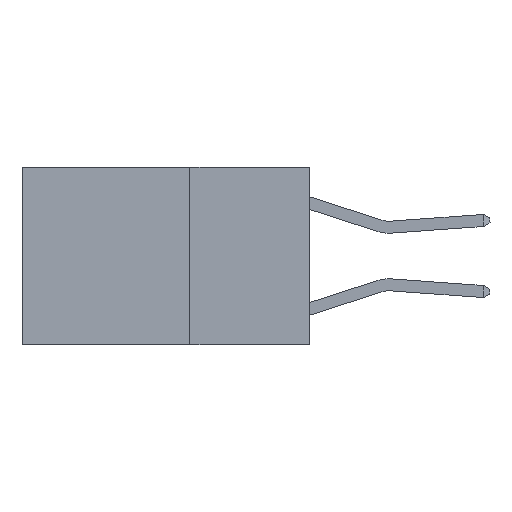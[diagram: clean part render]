
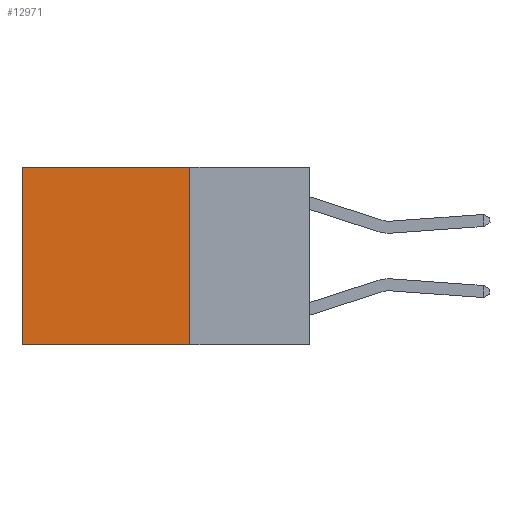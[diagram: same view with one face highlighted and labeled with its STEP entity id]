
A CAD part, left-side view. The second image highlights one B-rep face of the part: STEP entity #12971.
In plain terms, the highlighted planar face has unit normal (-1, 0, 0).
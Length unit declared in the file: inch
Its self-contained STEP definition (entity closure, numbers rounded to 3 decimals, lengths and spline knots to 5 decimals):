
#613 = VECTOR ( 'NONE', #1152, 39.37008 ) ;
#1152 = DIRECTION ( 'NONE',  ( 0., 1., 0. ) ) ;
#1472 = VECTOR ( 'NONE', #15156, 39.37008 ) ;
#1720 = DIRECTION ( 'NONE',  ( 1., 0., 0. ) ) ;
#2119 = VERTEX_POINT ( 'NONE', #9985 ) ;
#2372 = ORIENTED_EDGE ( 'NONE', *, *, #3028, .F. ) ;
#3028 = EDGE_CURVE ( 'NONE', #2119, #4737, #8661, .T. ) ;
#3346 = AXIS2_PLACEMENT_3D ( 'NONE', #12915, #1720, #12985 ) ;
#3936 = ORIENTED_EDGE ( 'NONE', *, *, #6628, .F. ) ;
#4737 = VERTEX_POINT ( 'NONE', #15641 ) ;
#5472 = CARTESIAN_POINT ( 'NONE',  ( 0.2625, 0.25, 0. ) ) ;
#5531 = VERTEX_POINT ( 'NONE', #11012 ) ;
#5959 = VECTOR ( 'NONE', #7079, 39.37008 ) ;
#6628 = EDGE_CURVE ( 'NONE', #10627, #2119, #14297, .T. ) ;
#7079 = DIRECTION ( 'NONE',  ( 0., 1., 0. ) ) ;
#8661 = LINE ( 'NONE', #12424, #613 ) ;
#8868 = EDGE_LOOP ( 'NONE', ( #12994, #2372, #3936, #12201 ) ) ;
#9985 = CARTESIAN_POINT ( 'NONE',  ( 0.2625, 0.25, -0.37 ) ) ;
#10627 = VERTEX_POINT ( 'NONE', #18249 ) ;
#10815 = CARTESIAN_POINT ( 'NONE',  ( 0.2625, 0.6, 0. ) ) ;
#11012 = CARTESIAN_POINT ( 'NONE',  ( 0.2625, 0.6, 0. ) ) ;
#12201 = ORIENTED_EDGE ( 'NONE', *, *, #16795, .T. ) ;
#12424 = CARTESIAN_POINT ( 'NONE',  ( 0.2625, 0.25, -0.37 ) ) ;
#12915 = CARTESIAN_POINT ( 'NONE',  ( 0.2625, 0.25, 0. ) ) ;
#12971 = ADVANCED_FACE ( 'NONE', ( #19591 ), #17740, .F. ) ;
#12985 = DIRECTION ( 'NONE',  ( 0., 0., -1. ) ) ;
#12994 = ORIENTED_EDGE ( 'NONE', *, *, #19085, .T. ) ;
#13569 = CARTESIAN_POINT ( 'NONE',  ( 0.2625, 0.25, 0. ) ) ;
#14297 = LINE ( 'NONE', #13569, #1472 ) ;
#14503 = LINE ( 'NONE', #5472, #5959 ) ;
#14902 = LINE ( 'NONE', #10815, #18164 ) ;
#15156 = DIRECTION ( 'NONE',  ( 0., 0., -1. ) ) ;
#15641 = CARTESIAN_POINT ( 'NONE',  ( 0.2625, 0.6, -0.37 ) ) ;
#16795 = EDGE_CURVE ( 'NONE', #10627, #5531, #14503, .T. ) ;
#17740 = PLANE ( 'NONE',  #3346 ) ;
#18164 = VECTOR ( 'NONE', #18769, 39.37008 ) ;
#18249 = CARTESIAN_POINT ( 'NONE',  ( 0.2625, 0.25, 0. ) ) ;
#18769 = DIRECTION ( 'NONE',  ( 0., 0., -1. ) ) ;
#19085 = EDGE_CURVE ( 'NONE', #5531, #4737, #14902, .T. ) ;
#19591 = FACE_OUTER_BOUND ( 'NONE', #8868, .T. ) ;
